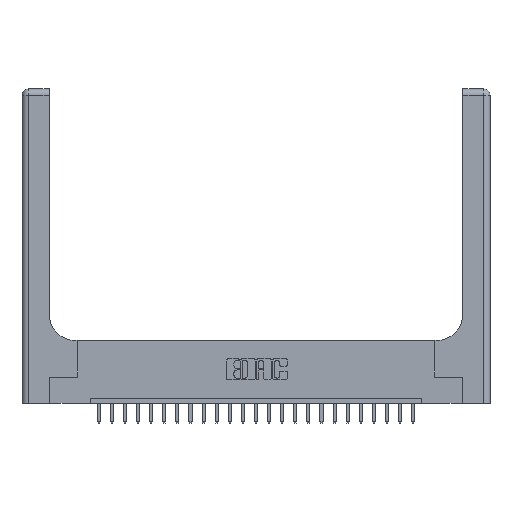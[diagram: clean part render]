
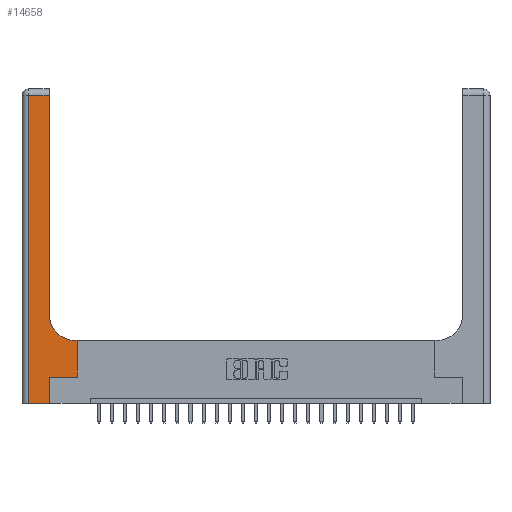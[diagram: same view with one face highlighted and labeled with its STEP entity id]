
A CAD part, top view. The second image highlights one B-rep face of the part: STEP entity #14658.
In plain terms, the highlighted planar face has unit normal (0, 0, 1).
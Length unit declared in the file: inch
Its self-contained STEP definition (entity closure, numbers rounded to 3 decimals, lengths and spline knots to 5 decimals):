
#34 = CARTESIAN_POINT ( 'NONE',  ( 0.528, 0.6, 0.37 ) ) ;
#232 = CARTESIAN_POINT ( 'NONE',  ( 0.265, 0., 0.37 ) ) ;
#408 = LINE ( 'NONE', #18515, #19447 ) ;
#476 = DIRECTION ( 'NONE',  ( 1., 0., 0. ) ) ;
#499 = CARTESIAN_POINT ( 'NONE',  ( 0.06, 2.94, 0.37 ) ) ;
#792 = EDGE_CURVE ( 'NONE', #17548, #2607, #20186, .T. ) ;
#875 = DIRECTION ( 'NONE',  ( 0., -1., 0. ) ) ;
#1079 = ORIENTED_EDGE ( 'NONE', *, *, #792, .T. ) ;
#1096 = EDGE_CURVE ( 'NONE', #7880, #7993, #11068, .T. ) ;
#1352 = DIRECTION ( 'NONE',  ( -1., 0., 0. ) ) ;
#1398 = VERTEX_POINT ( 'NONE', #15550 ) ;
#1722 = EDGE_CURVE ( 'NONE', #3585, #17548, #408, .T. ) ;
#2380 = CARTESIAN_POINT ( 'NONE',  ( 0.06, 0., 0.37 ) ) ;
#2607 = VERTEX_POINT ( 'NONE', #11392 ) ;
#3566 = DIRECTION ( 'NONE',  ( -1., 0., 0. ) ) ;
#3585 = VERTEX_POINT ( 'NONE', #499 ) ;
#3690 = CARTESIAN_POINT ( 'NONE',  ( 0.51, 0.6, 0.37 ) ) ;
#4140 = VECTOR ( 'NONE', #22522, 39.37008 ) ;
#4505 = DIRECTION ( 'NONE',  ( 0., 0., -1. ) ) ;
#4880 = EDGE_CURVE ( 'NONE', #7993, #1398, #8113, .T. ) ;
#5249 = CARTESIAN_POINT ( 'NONE',  ( 0.26, 0.6, 0.37 ) ) ;
#5463 = LINE ( 'NONE', #20236, #17680 ) ;
#5880 = EDGE_CURVE ( 'NONE', #18993, #20963, #17540, .T. ) ;
#6531 = EDGE_CURVE ( 'NONE', #1398, #3585, #5463, .T. ) ;
#6697 = CARTESIAN_POINT ( 'NONE',  ( 0.265, 0.25, 0.37 ) ) ;
#7306 = CARTESIAN_POINT ( 'NONE',  ( 0.528, 0.25, 0.37 ) ) ;
#7464 = LINE ( 'NONE', #232, #10334 ) ;
#7466 = VERTEX_POINT ( 'NONE', #34 ) ;
#7760 = DIRECTION ( 'NONE',  ( 0., 1., 0. ) ) ;
#7822 = DIRECTION ( 'NONE',  ( 0., 1., 0. ) ) ;
#7880 = VERTEX_POINT ( 'NONE', #3690 ) ;
#7974 = ORIENTED_EDGE ( 'NONE', *, *, #1722, .T. ) ;
#7993 = VERTEX_POINT ( 'NONE', #22490 ) ;
#8113 = LINE ( 'NONE', #15397, #19330 ) ;
#8941 = DIRECTION ( 'NONE',  ( -1., 0., 0. ) ) ;
#9627 = CARTESIAN_POINT ( 'NONE',  ( 0.51, 0.85, 0.37 ) ) ;
#10334 = VECTOR ( 'NONE', #7822, 39.37008 ) ;
#10385 = DIRECTION ( 'NONE',  ( 0., 0., -1. ) ) ;
#10779 = LINE ( 'NONE', #7306, #19311 ) ;
#11068 = CIRCLE ( 'NONE', #14118, 0.25 ) ;
#11392 = CARTESIAN_POINT ( 'NONE',  ( 0.265, 0., 0.37 ) ) ;
#12243 = VECTOR ( 'NONE', #8941, 39.37008 ) ;
#12505 = ORIENTED_EDGE ( 'NONE', *, *, #1096, .T. ) ;
#12536 = EDGE_CURVE ( 'NONE', #20963, #7466, #10779, .T. ) ;
#12577 = DIRECTION ( 'NONE',  ( 0., 1., 0. ) ) ;
#13579 = CARTESIAN_POINT ( 'NONE',  ( 0.265, 0.25, 0.37 ) ) ;
#13852 = PLANE ( 'NONE',  #19763 ) ;
#14118 = AXIS2_PLACEMENT_3D ( 'NONE', #9627, #4505, #476 ) ;
#14315 = LINE ( 'NONE', #5249, #12243 ) ;
#14658 = ADVANCED_FACE ( 'NONE', ( #19327 ), #13852, .F. ) ;
#14720 = EDGE_LOOP ( 'NONE', ( #19346, #18123, #7974, #1079, #21937, #23426, #23390, #19865, #12505 ) ) ;
#15397 = CARTESIAN_POINT ( 'NONE',  ( 0.26, 3., 0.37 ) ) ;
#15550 = CARTESIAN_POINT ( 'NONE',  ( 0.26, 2.94, 0.37 ) ) ;
#15644 = DIRECTION ( 'NONE',  ( 1., 0., 0. ) ) ;
#17540 = LINE ( 'NONE', #6697, #21678 ) ;
#17548 = VERTEX_POINT ( 'NONE', #2380 ) ;
#17680 = VECTOR ( 'NONE', #3566, 39.37008 ) ;
#18123 = ORIENTED_EDGE ( 'NONE', *, *, #6531, .T. ) ;
#18515 = CARTESIAN_POINT ( 'NONE',  ( 0.06, 3., 0.37 ) ) ;
#18806 = EDGE_CURVE ( 'NONE', #7466, #7880, #14315, .T. ) ;
#18951 = CARTESIAN_POINT ( 'NONE',  ( 0., 0., 0.37 ) ) ;
#18993 = VERTEX_POINT ( 'NONE', #13579 ) ;
#19181 = EDGE_CURVE ( 'NONE', #2607, #18993, #7464, .T. ) ;
#19209 = CARTESIAN_POINT ( 'NONE',  ( 0., 3., 0.37 ) ) ;
#19235 = CARTESIAN_POINT ( 'NONE',  ( 0.528, 0.25, 0.37 ) ) ;
#19311 = VECTOR ( 'NONE', #12577, 39.37008 ) ;
#19327 = FACE_OUTER_BOUND ( 'NONE', #14720, .T. ) ;
#19330 = VECTOR ( 'NONE', #7760, 39.37008 ) ;
#19346 = ORIENTED_EDGE ( 'NONE', *, *, #4880, .T. ) ;
#19447 = VECTOR ( 'NONE', #875, 39.37008 ) ;
#19763 = AXIS2_PLACEMENT_3D ( 'NONE', #19209, #10385, #1352 ) ;
#19865 = ORIENTED_EDGE ( 'NONE', *, *, #18806, .T. ) ;
#20186 = LINE ( 'NONE', #18951, #4140 ) ;
#20236 = CARTESIAN_POINT ( 'NONE',  ( 0., 2.94, 0.37 ) ) ;
#20963 = VERTEX_POINT ( 'NONE', #19235 ) ;
#21678 = VECTOR ( 'NONE', #15644, 39.37008 ) ;
#21937 = ORIENTED_EDGE ( 'NONE', *, *, #19181, .T. ) ;
#22490 = CARTESIAN_POINT ( 'NONE',  ( 0.26, 0.85, 0.37 ) ) ;
#22522 = DIRECTION ( 'NONE',  ( 1., 0., 0. ) ) ;
#23390 = ORIENTED_EDGE ( 'NONE', *, *, #12536, .T. ) ;
#23426 = ORIENTED_EDGE ( 'NONE', *, *, #5880, .T. ) ;
